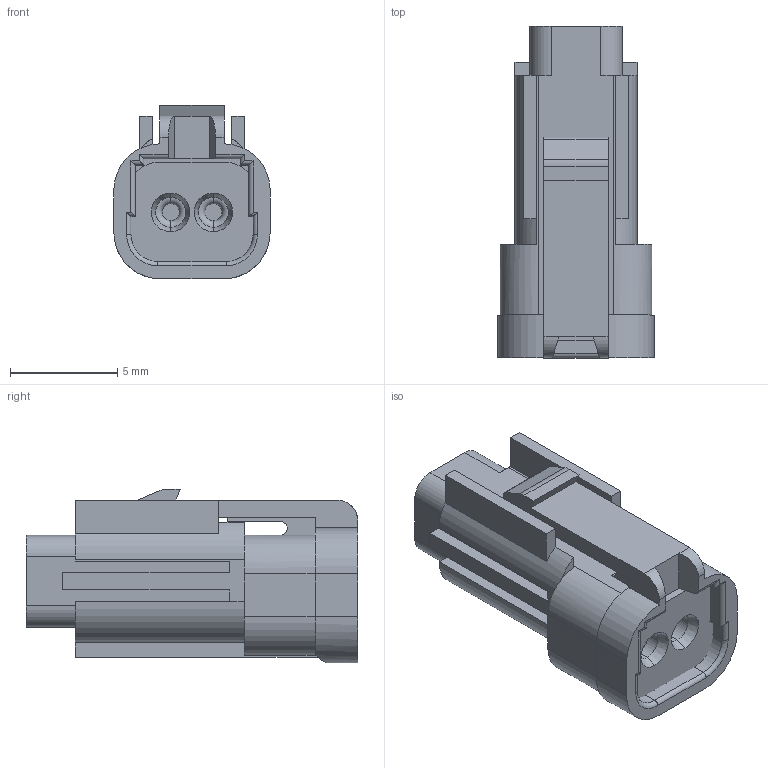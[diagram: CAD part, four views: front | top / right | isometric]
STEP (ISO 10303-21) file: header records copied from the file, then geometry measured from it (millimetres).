
FILE_DESCRIPTION (( 'STEP AP203' ), '1' );
FILE_NAME ('566-002-000-810.STEP', '2021-09-21T14:21:54', ( '' ), ( '' ), 'SwSTEP 2.0', 'SolidWorks 2020', '' );
FILE_SCHEMA (( 'CONFIG_CONTROL_DESIGN' ));
Length unit declared in the file: millimetre
Products named in the file (1): 566-002-000-810
Bounding box: 7.3 x 15.5 x 8.1 mm (x, y, z)
Volume: 439.3 mm3; surface area: 915.9 mm2
Topology: 2 solids, 2 shells, 364 faces, 930 edges, 574 vertices
Faces by surface type: plane 226, cylinder 80, torus 46, cone 12
Entity records: 11051 total; most frequent: CARTESIAN_POINT 2133, ORIENTED_EDGE 1860, DIRECTION 1822, EDGE_CURVE 930, VECTOR 688, LINE 688, VERTEX_POINT 574, AXIS2_PLACEMENT_3D 567
